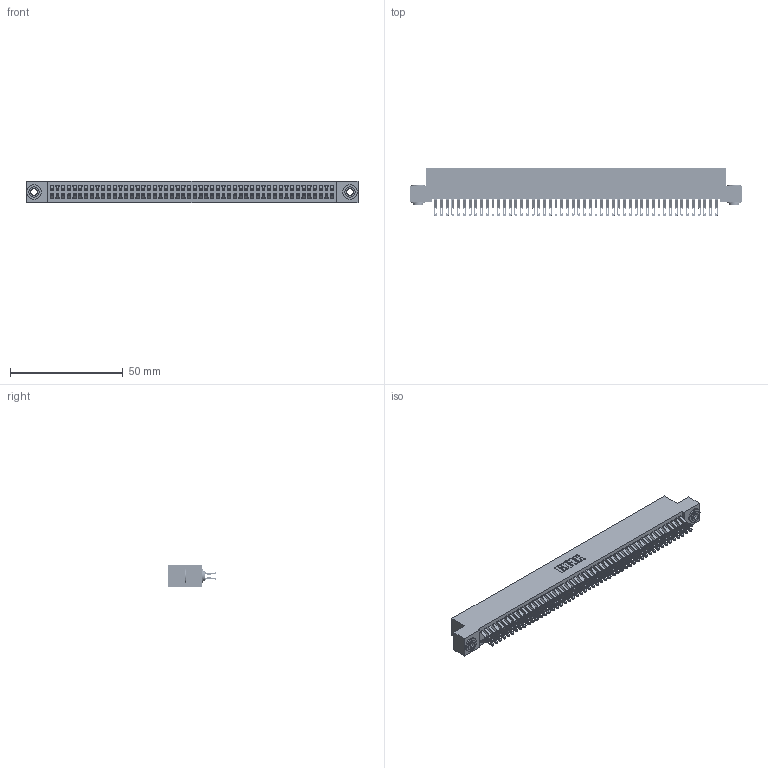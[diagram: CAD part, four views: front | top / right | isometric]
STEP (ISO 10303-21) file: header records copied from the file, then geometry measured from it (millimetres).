
FILE_DESCRIPTION (( 'STEP AP203' ), '1' );
FILE_NAME ('342-100-555-203.STEP', '2019-10-04T17:47:04', ( '' ), ( '' ), 'SwSTEP 2.0', 'SolidWorks 2016', '' );
FILE_SCHEMA (( 'CONFIG_CONTROL_DESIGN' ));
Length unit declared in the file: inch
Products named in the file (4): 342 Part_.156 TH; 345-292-001_555 Tail; 342-250-002_345-250-002-102; 342-100-555-203
Assembly tree (103 placements, depth 2):
  342-100-555-203
    342 Part_.156 TH
    345-292-001_555 Tail  x100
    342-250-002_345-250-002-102  x2
Bounding box: 147.32 x 21.47 x 9.4 mm (x, y, z)
Volume: 13575.3 mm3; surface area: 23475.9 mm2
Topology: 103 solids, 103 shells, 5948 faces, 18675 edges, 12446 vertices
Faces by surface type: plane 3476, cylinder 2464, cone 8
Entity records: 31976 total; most frequent: CARTESIAN_POINT 5299, ORIENTED_EDGE 5198, DIRECTION 4517, EDGE_CURVE 2599, VECTOR 2427, LINE 2427, VERTEX_POINT 1730, AXIS2_PLACEMENT_3D 1045
